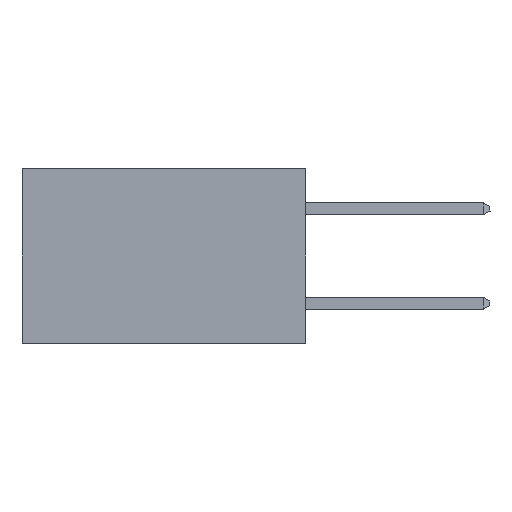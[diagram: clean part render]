
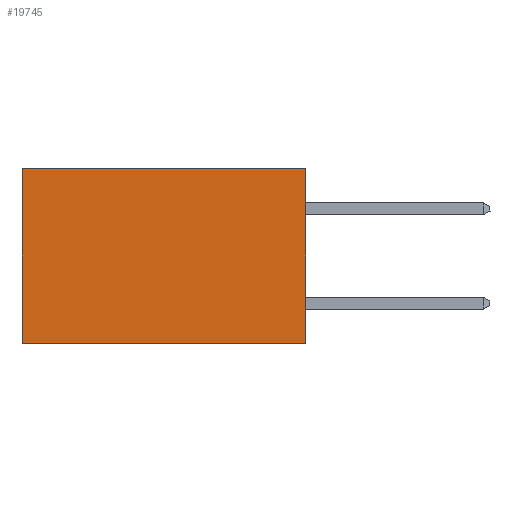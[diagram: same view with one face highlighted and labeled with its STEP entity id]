
A CAD part, left-side view. The second image highlights one B-rep face of the part: STEP entity #19745.
In plain terms, the highlighted planar face has unit normal (-1, 0, 0).
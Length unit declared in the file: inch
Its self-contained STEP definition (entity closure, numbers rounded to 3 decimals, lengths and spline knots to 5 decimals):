
#245 = DIRECTION ( 'NONE',  ( 0., 0., -1. ) ) ;
#525 = EDGE_CURVE ( 'NONE', #13774, #25827, #17481, .T. ) ;
#576 = DIRECTION ( 'NONE',  ( 0., 1., 0. ) ) ;
#1421 = CARTESIAN_POINT ( 'NONE',  ( 0.298, 0., 0. ) ) ;
#1657 = AXIS2_PLACEMENT_3D ( 'NONE', #18091, #6098, #16166 ) ;
#1975 = VERTEX_POINT ( 'NONE', #14968 ) ;
#1983 = VECTOR ( 'NONE', #18062, 39.37008 ) ;
#2085 = CARTESIAN_POINT ( 'NONE',  ( 0.298, 0., 0. ) ) ;
#2390 = DIRECTION ( 'NONE',  ( 0., 0., -1. ) ) ;
#2832 = EDGE_CURVE ( 'NONE', #21829, #13774, #12327, .T. ) ;
#2834 = EDGE_CURVE ( 'NONE', #1975, #25827, #11099, .T. ) ;
#3836 = EDGE_CURVE ( 'NONE', #21829, #1975, #12584, .T. ) ;
#4437 = CARTESIAN_POINT ( 'NONE',  ( 0.298, 0., -0.37 ) ) ;
#5755 = VECTOR ( 'NONE', #245, 39.37008 ) ;
#6098 = DIRECTION ( 'NONE',  ( 1., 0., 0. ) ) ;
#8398 = CARTESIAN_POINT ( 'NONE',  ( 0.298, 0.6, 0. ) ) ;
#10776 = CARTESIAN_POINT ( 'NONE',  ( 0.298, 0., -0.37 ) ) ;
#11099 = LINE ( 'NONE', #8398, #5755 ) ;
#12327 = LINE ( 'NONE', #22223, #21739 ) ;
#12537 = ORIENTED_EDGE ( 'NONE', *, *, #3836, .T. ) ;
#12584 = LINE ( 'NONE', #2085, #1983 ) ;
#13774 = VERTEX_POINT ( 'NONE', #10776 ) ;
#14968 = CARTESIAN_POINT ( 'NONE',  ( 0.298, 0.6, 0. ) ) ;
#16066 = PLANE ( 'NONE',  #1657 ) ;
#16166 = DIRECTION ( 'NONE',  ( 0., 0., -1. ) ) ;
#16747 = CARTESIAN_POINT ( 'NONE',  ( 0.298, 0.6, -0.37 ) ) ;
#17481 = LINE ( 'NONE', #4437, #17798 ) ;
#17798 = VECTOR ( 'NONE', #576, 39.37008 ) ;
#18062 = DIRECTION ( 'NONE',  ( 0., 1., 0. ) ) ;
#18091 = CARTESIAN_POINT ( 'NONE',  ( 0.298, 0., 0. ) ) ;
#19745 = ADVANCED_FACE ( 'NONE', ( #21620 ), #16066, .F. ) ;
#19914 = ORIENTED_EDGE ( 'NONE', *, *, #2834, .T. ) ;
#21620 = FACE_OUTER_BOUND ( 'NONE', #23760, .T. ) ;
#21682 = ORIENTED_EDGE ( 'NONE', *, *, #525, .F. ) ;
#21739 = VECTOR ( 'NONE', #2390, 39.37008 ) ;
#21829 = VERTEX_POINT ( 'NONE', #1421 ) ;
#22223 = CARTESIAN_POINT ( 'NONE',  ( 0.298, 0., 0. ) ) ;
#22866 = ORIENTED_EDGE ( 'NONE', *, *, #2832, .F. ) ;
#23760 = EDGE_LOOP ( 'NONE', ( #19914, #21682, #22866, #12537 ) ) ;
#25827 = VERTEX_POINT ( 'NONE', #16747 ) ;
